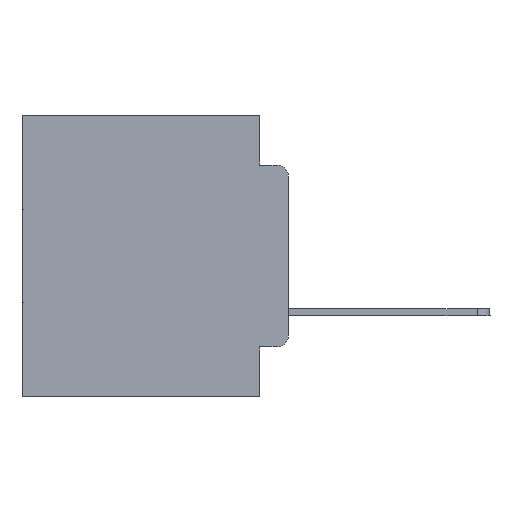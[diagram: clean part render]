
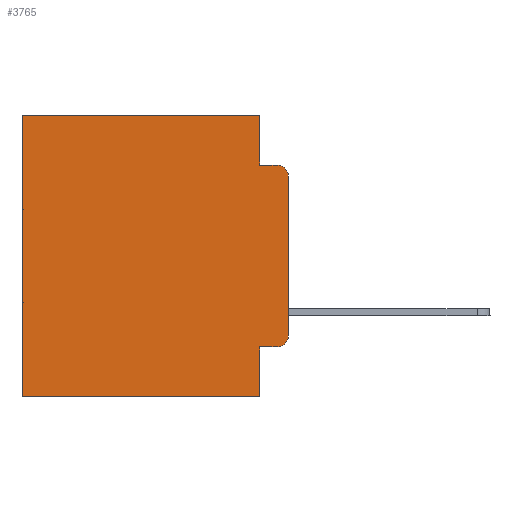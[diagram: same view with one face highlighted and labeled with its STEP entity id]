
A CAD part, left-side view. The second image highlights one B-rep face of the part: STEP entity #3765.
In plain terms, the highlighted planar face has unit normal (-1, 0, 0).
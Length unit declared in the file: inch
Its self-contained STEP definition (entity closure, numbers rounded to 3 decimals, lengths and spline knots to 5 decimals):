
#183 = EDGE_CURVE ( 'NONE', #11110, #29578, #26146, .T. ) ;
#513 = VECTOR ( 'NONE', #21481, 39.37008 ) ;
#2346 = ORIENTED_EDGE ( 'NONE', *, *, #28366, .T. ) ;
#2926 = CARTESIAN_POINT ( 'NONE',  ( 0.298, 0.051, 0. ) ) ;
#3126 = CARTESIAN_POINT ( 'NONE',  ( 0.298, 0., 0. ) ) ;
#3131 = EDGE_CURVE ( 'NONE', #18673, #12512, #6178, .T. ) ;
#3369 = CARTESIAN_POINT ( 'NONE',  ( 0.298, 0.473, -0.5 ) ) ;
#3538 = CARTESIAN_POINT ( 'NONE',  ( 0.298, 0.02, -0.0885 ) ) ;
#3765 = ADVANCED_FACE ( 'NONE', ( #28119 ), #23087, .F. ) ;
#4858 = AXIS2_PLACEMENT_3D ( 'NONE', #9284, #6851, #25393 ) ;
#5084 = VECTOR ( 'NONE', #24629, 39.37008 ) ;
#5617 = CIRCLE ( 'NONE', #22909, 0.02 ) ;
#6007 = VECTOR ( 'NONE', #12040, 39.37008 ) ;
#6178 = LINE ( 'NONE', #26836, #5084 ) ;
#6210 = ORIENTED_EDGE ( 'NONE', *, *, #3131, .T. ) ;
#6851 = DIRECTION ( 'NONE',  ( 1., 0., 0. ) ) ;
#6943 = VERTEX_POINT ( 'NONE', #10650 ) ;
#7167 = VERTEX_POINT ( 'NONE', #13363 ) ;
#8550 = LINE ( 'NONE', #10296, #26168 ) ;
#8570 = CARTESIAN_POINT ( 'NONE',  ( 0.298, 0.051, -0.5 ) ) ;
#8581 = CARTESIAN_POINT ( 'NONE',  ( 0.298, 0., -0.3915 ) ) ;
#8589 = DIRECTION ( 'NONE',  ( 0., 1., 0. ) ) ;
#8595 = VERTEX_POINT ( 'NONE', #17703 ) ;
#8743 = EDGE_CURVE ( 'NONE', #8595, #24408, #26541, .T. ) ;
#9284 = CARTESIAN_POINT ( 'NONE',  ( 0.298, 0., 0. ) ) ;
#9292 = EDGE_CURVE ( 'NONE', #23417, #29578, #18568, .T. ) ;
#10296 = CARTESIAN_POINT ( 'NONE',  ( 0.298, 0.051, 0. ) ) ;
#10433 = DIRECTION ( 'NONE',  ( 0., 0., -1. ) ) ;
#10650 = CARTESIAN_POINT ( 'NONE',  ( 0.298, 0.051, 0. ) ) ;
#10792 = DIRECTION ( 'NONE',  ( 0., 0., -1. ) ) ;
#11110 = VERTEX_POINT ( 'NONE', #19322 ) ;
#11374 = LINE ( 'NONE', #2926, #513 ) ;
#11446 = VECTOR ( 'NONE', #23409, 39.37008 ) ;
#12040 = DIRECTION ( 'NONE',  ( 0., 1., 0. ) ) ;
#12512 = VERTEX_POINT ( 'NONE', #23740 ) ;
#12534 = EDGE_LOOP ( 'NONE', ( #14894, #19790, #13198, #29482, #2346, #18597, #24042, #29315, #6210, #16141 ) ) ;
#12914 = CARTESIAN_POINT ( 'NONE',  ( 0.298, 0.02, -0.3915 ) ) ;
#13069 = EDGE_CURVE ( 'NONE', #12512, #21477, #5617, .T. ) ;
#13198 = ORIENTED_EDGE ( 'NONE', *, *, #13609, .F. ) ;
#13227 = VECTOR ( 'NONE', #18587, 39.37008 ) ;
#13252 = EDGE_CURVE ( 'NONE', #8595, #21477, #15006, .T. ) ;
#13363 = CARTESIAN_POINT ( 'NONE',  ( 0.298, 0.051, -0.0885 ) ) ;
#13533 = EDGE_CURVE ( 'NONE', #18673, #23417, #8550, .T. ) ;
#13608 = DIRECTION ( 'NONE',  ( 0., 0., -1. ) ) ;
#13609 = EDGE_CURVE ( 'NONE', #7167, #24408, #19291, .T. ) ;
#14894 = ORIENTED_EDGE ( 'NONE', *, *, #13252, .F. ) ;
#15006 = LINE ( 'NONE', #26345, #18227 ) ;
#15522 = DIRECTION ( 'NONE',  ( -1., 0., 0. ) ) ;
#16141 = ORIENTED_EDGE ( 'NONE', *, *, #13069, .T. ) ;
#16347 = CARTESIAN_POINT ( 'NONE',  ( 0.298, 0.051, -0.4115 ) ) ;
#16521 = EDGE_CURVE ( 'NONE', #6943, #7167, #11374, .T. ) ;
#16737 = AXIS2_PLACEMENT_3D ( 'NONE', #27346, #25058, #13608 ) ;
#17703 = CARTESIAN_POINT ( 'NONE',  ( 0.298, 0., -0.1085 ) ) ;
#17931 = CARTESIAN_POINT ( 'NONE',  ( 0.298, 0., -0.5 ) ) ;
#18227 = VECTOR ( 'NONE', #10433, 39.37008 ) ;
#18568 = LINE ( 'NONE', #17931, #21087 ) ;
#18587 = DIRECTION ( 'NONE',  ( 0., 0., -1. ) ) ;
#18597 = ORIENTED_EDGE ( 'NONE', *, *, #183, .T. ) ;
#18673 = VERTEX_POINT ( 'NONE', #16347 ) ;
#18962 = CARTESIAN_POINT ( 'NONE',  ( 0.298, 0.051, -0.0885 ) ) ;
#19291 = LINE ( 'NONE', #18962, #11446 ) ;
#19322 = CARTESIAN_POINT ( 'NONE',  ( 0.298, 0.473, 0. ) ) ;
#19661 = DIRECTION ( 'NONE',  ( 0., 0., -1. ) ) ;
#19790 = ORIENTED_EDGE ( 'NONE', *, *, #8743, .T. ) ;
#21087 = VECTOR ( 'NONE', #8589, 39.37008 ) ;
#21477 = VERTEX_POINT ( 'NONE', #8581 ) ;
#21481 = DIRECTION ( 'NONE',  ( 0., 0., -1. ) ) ;
#22909 = AXIS2_PLACEMENT_3D ( 'NONE', #12914, #15522, #10792 ) ;
#23087 = PLANE ( 'NONE',  #4858 ) ;
#23409 = DIRECTION ( 'NONE',  ( 0., -1., 0. ) ) ;
#23417 = VERTEX_POINT ( 'NONE', #8570 ) ;
#23740 = CARTESIAN_POINT ( 'NONE',  ( 0.298, 0.02, -0.4115 ) ) ;
#24042 = ORIENTED_EDGE ( 'NONE', *, *, #9292, .F. ) ;
#24408 = VERTEX_POINT ( 'NONE', #3538 ) ;
#24629 = DIRECTION ( 'NONE',  ( 0., -1., 0. ) ) ;
#25058 = DIRECTION ( 'NONE',  ( -1., 0., 0. ) ) ;
#25351 = CARTESIAN_POINT ( 'NONE',  ( 0.298, 0.473, 0. ) ) ;
#25393 = DIRECTION ( 'NONE',  ( 0., 0., -1. ) ) ;
#25827 = LINE ( 'NONE', #3126, #6007 ) ;
#26146 = LINE ( 'NONE', #25351, #13227 ) ;
#26168 = VECTOR ( 'NONE', #19661, 39.37008 ) ;
#26345 = CARTESIAN_POINT ( 'NONE',  ( 0.298, 0., 0. ) ) ;
#26541 = CIRCLE ( 'NONE', #16737, 0.02 ) ;
#26836 = CARTESIAN_POINT ( 'NONE',  ( 0.298, 0.051, -0.4115 ) ) ;
#27346 = CARTESIAN_POINT ( 'NONE',  ( 0.298, 0.02, -0.1085 ) ) ;
#28119 = FACE_OUTER_BOUND ( 'NONE', #12534, .T. ) ;
#28366 = EDGE_CURVE ( 'NONE', #6943, #11110, #25827, .T. ) ;
#29315 = ORIENTED_EDGE ( 'NONE', *, *, #13533, .F. ) ;
#29482 = ORIENTED_EDGE ( 'NONE', *, *, #16521, .F. ) ;
#29578 = VERTEX_POINT ( 'NONE', #3369 ) ;
